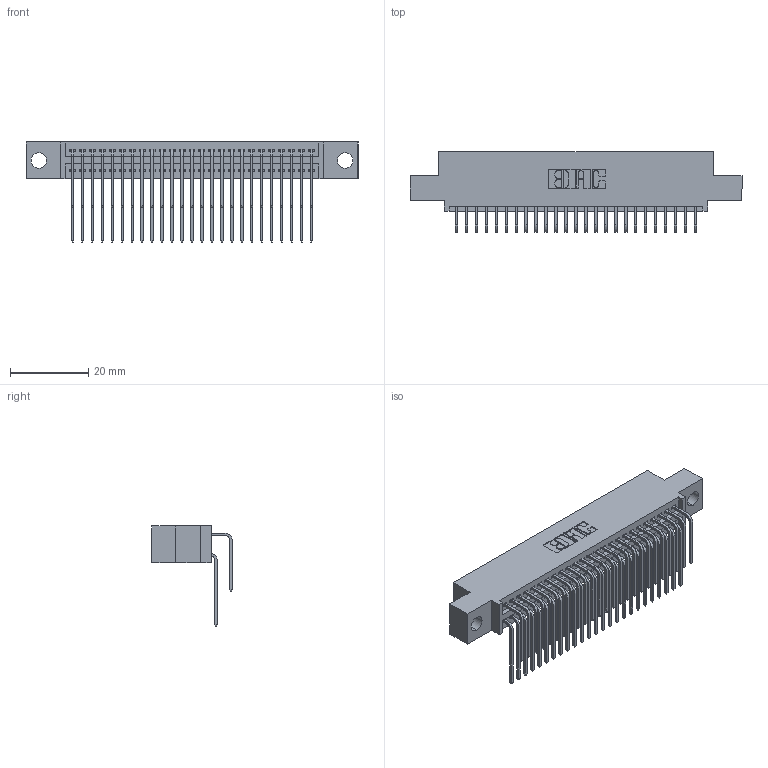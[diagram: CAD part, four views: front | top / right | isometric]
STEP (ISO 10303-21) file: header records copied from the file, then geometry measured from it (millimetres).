
FILE_DESCRIPTION (( 'STEP AP203' ), '1' );
FILE_NAME ('395-050-559-504.STEP', '2021-06-17T00:05:13', ( '' ), ( '' ), 'SwSTEP 2.0', 'SolidWorks 2020', '' );
FILE_SCHEMA (( 'CONFIG_CONTROL_DESIGN' ));
Length unit declared in the file: inch
Products named in the file (4): 345 Part_0.110 Offset - 0.156 Dia-TI; 345-292-001_558 559 Tail - 1; 345-292-001_559 Tail - 2; 395-050-559-504
Assembly tree (51 placements, depth 2):
  395-050-559-504
    345 Part_0.110 Offset - 0.156 Dia-TI
    345-292-001_558 559 Tail - 1  x25
    345-292-001_559 Tail - 2  x25
Bounding box: 84.71 x 20.56 x 25.53 mm (x, y, z)
Volume: 8180 mm3; surface area: 13063 mm2
Topology: 51 solids, 51 shells, 2744 faces, 8139 edges, 5358 vertices
Faces by surface type: plane 1848, cylinder 896
Entity records: 24107 total; most frequent: CARTESIAN_POINT 4109, ORIENTED_EDGE 3990, DIRECTION 3615, EDGE_CURVE 1995, LINE 1723, VECTOR 1723, VERTEX_POINT 1326, AXIS2_PLACEMENT_3D 946
